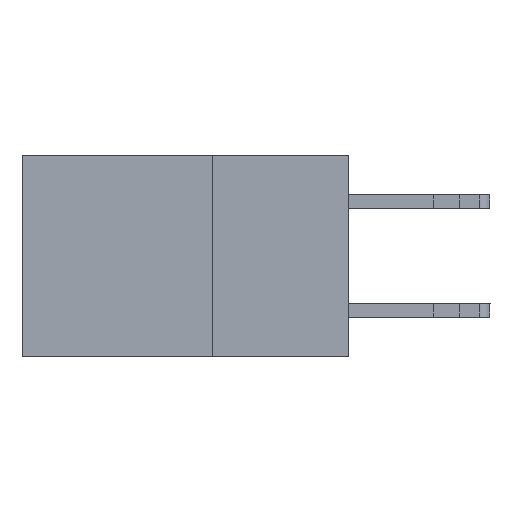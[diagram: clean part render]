
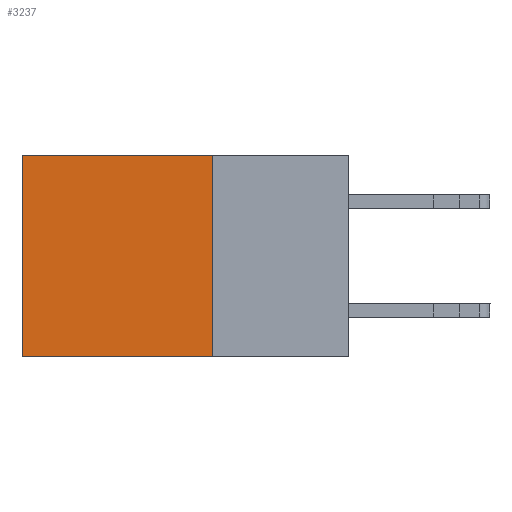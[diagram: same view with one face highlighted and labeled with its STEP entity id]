
A CAD part, left-side view. The second image highlights one B-rep face of the part: STEP entity #3237.
In plain terms, the highlighted planar face has unit normal (-1, 0, 0).
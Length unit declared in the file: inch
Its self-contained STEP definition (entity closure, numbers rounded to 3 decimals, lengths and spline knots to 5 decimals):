
#457 = ORIENTED_EDGE ( 'NONE', *, *, #1934, .F. ) ;
#482 = EDGE_LOOP ( 'NONE', ( #17626, #457, #10681, #19077 ) ) ;
#483 = CARTESIAN_POINT ( 'NONE',  ( 0.298, 0.25, -0.37 ) ) ;
#1934 = EDGE_CURVE ( 'NONE', #23374, #6492, #18439, .T. ) ;
#2828 = CARTESIAN_POINT ( 'NONE',  ( 0.298, 0.6, -0.37 ) ) ;
#2882 = VECTOR ( 'NONE', #23915, 39.37008 ) ;
#3237 = ADVANCED_FACE ( 'NONE', ( #15684 ), #16692, .F. ) ;
#6307 = AXIS2_PLACEMENT_3D ( 'NONE', #14519, #6863, #8797 ) ;
#6492 = VERTEX_POINT ( 'NONE', #2828 ) ;
#6552 = LINE ( 'NONE', #18443, #18270 ) ;
#6863 = DIRECTION ( 'NONE',  ( 1., 0., 0. ) ) ;
#7131 = DIRECTION ( 'NONE',  ( 0., 0., -1. ) ) ;
#8796 = CARTESIAN_POINT ( 'NONE',  ( 0.298, 0.25, 0. ) ) ;
#8797 = DIRECTION ( 'NONE',  ( 0., 0., -1. ) ) ;
#9446 = CARTESIAN_POINT ( 'NONE',  ( 0.298, 0.25, -0.37 ) ) ;
#9749 = VECTOR ( 'NONE', #10294, 39.37008 ) ;
#10294 = DIRECTION ( 'NONE',  ( 0., 1., 0. ) ) ;
#10328 = LINE ( 'NONE', #8796, #2882 ) ;
#10681 = ORIENTED_EDGE ( 'NONE', *, *, #23775, .F. ) ;
#11335 = LINE ( 'NONE', #17794, #16138 ) ;
#11829 = EDGE_CURVE ( 'NONE', #21356, #6492, #6552, .T. ) ;
#14123 = DIRECTION ( 'NONE',  ( 0., 0., -1. ) ) ;
#14519 = CARTESIAN_POINT ( 'NONE',  ( 0.298, 0.25, 0. ) ) ;
#15684 = FACE_OUTER_BOUND ( 'NONE', #482, .T. ) ;
#16138 = VECTOR ( 'NONE', #14123, 39.37008 ) ;
#16692 = PLANE ( 'NONE',  #6307 ) ;
#16859 = CARTESIAN_POINT ( 'NONE',  ( 0.298, 0.25, 0. ) ) ;
#17626 = ORIENTED_EDGE ( 'NONE', *, *, #11829, .T. ) ;
#17794 = CARTESIAN_POINT ( 'NONE',  ( 0.298, 0.25, 0. ) ) ;
#18270 = VECTOR ( 'NONE', #7131, 39.37008 ) ;
#18439 = LINE ( 'NONE', #483, #9749 ) ;
#18443 = CARTESIAN_POINT ( 'NONE',  ( 0.298, 0.6, 0. ) ) ;
#18967 = EDGE_CURVE ( 'NONE', #19196, #21356, #10328, .T. ) ;
#19077 = ORIENTED_EDGE ( 'NONE', *, *, #18967, .T. ) ;
#19196 = VERTEX_POINT ( 'NONE', #16859 ) ;
#21356 = VERTEX_POINT ( 'NONE', #21995 ) ;
#21995 = CARTESIAN_POINT ( 'NONE',  ( 0.298, 0.6, 0. ) ) ;
#23374 = VERTEX_POINT ( 'NONE', #9446 ) ;
#23775 = EDGE_CURVE ( 'NONE', #19196, #23374, #11335, .T. ) ;
#23915 = DIRECTION ( 'NONE',  ( 0., 1., 0. ) ) ;
